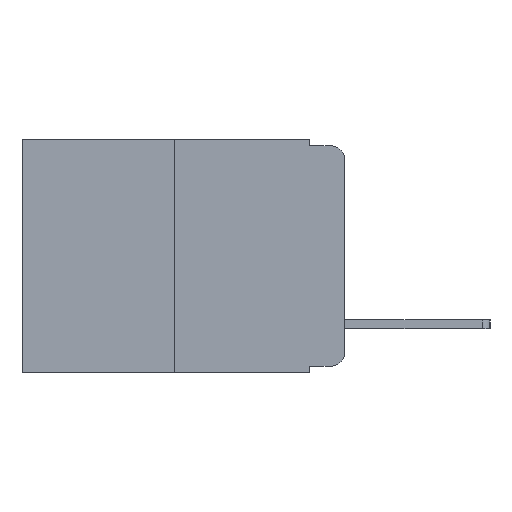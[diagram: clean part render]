
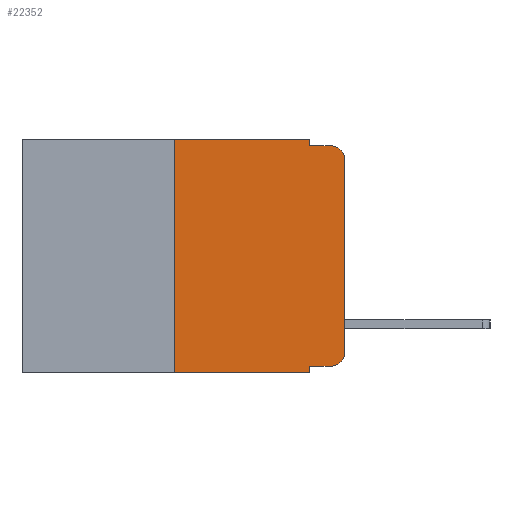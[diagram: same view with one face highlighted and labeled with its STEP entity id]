
A CAD part, left-side view. The second image highlights one B-rep face of the part: STEP entity #22352.
In plain terms, the highlighted planar face has unit normal (-1, 0, 0).
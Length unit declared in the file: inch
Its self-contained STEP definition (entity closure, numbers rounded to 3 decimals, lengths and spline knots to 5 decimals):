
#346 = CARTESIAN_POINT ( 'NONE',  ( 0., 0.051, -0.333 ) ) ;
#444 = CARTESIAN_POINT ( 'NONE',  ( 0., 0.02, -0.313 ) ) ;
#696 = EDGE_CURVE ( 'NONE', #20087, #22232, #1497, .T. ) ;
#750 = VERTEX_POINT ( 'NONE', #14333 ) ;
#879 = EDGE_CURVE ( 'NONE', #14549, #750, #12049, .T. ) ;
#1497 = LINE ( 'NONE', #20543, #21578 ) ;
#1663 = CARTESIAN_POINT ( 'NONE',  ( 0., 0.051, -0.01 ) ) ;
#2010 = EDGE_CURVE ( 'NONE', #13390, #22232, #22094, .T. ) ;
#2052 = VECTOR ( 'NONE', #11614, 39.37008 ) ;
#2058 = LINE ( 'NONE', #346, #11725 ) ;
#2358 = EDGE_CURVE ( 'NONE', #5249, #17747, #18879, .T. ) ;
#2439 = DIRECTION ( 'NONE',  ( 0., 0., -1. ) ) ;
#2460 = CARTESIAN_POINT ( 'NONE',  ( 0., 0.02, -0.03 ) ) ;
#3865 = DIRECTION ( 'NONE',  ( 0., -1., 0. ) ) ;
#4219 = ORIENTED_EDGE ( 'NONE', *, *, #10292, .T. ) ;
#4291 = ORIENTED_EDGE ( 'NONE', *, *, #14017, .T. ) ;
#4403 = DIRECTION ( 'NONE',  ( 0., -1., 0. ) ) ;
#4554 = CARTESIAN_POINT ( 'NONE',  ( 0., 0.051, -0.333 ) ) ;
#4584 = ORIENTED_EDGE ( 'NONE', *, *, #15250, .F. ) ;
#4840 = PLANE ( 'NONE',  #10993 ) ;
#5046 = VERTEX_POINT ( 'NONE', #6296 ) ;
#5072 = ORIENTED_EDGE ( 'NONE', *, *, #2358, .T. ) ;
#5108 = VECTOR ( 'NONE', #3865, 39.37008 ) ;
#5249 = VERTEX_POINT ( 'NONE', #21710 ) ;
#5967 = EDGE_CURVE ( 'NONE', #5046, #13390, #11704, .T. ) ;
#6157 = CARTESIAN_POINT ( 'NONE',  ( 0., 0.051, 0. ) ) ;
#6296 = CARTESIAN_POINT ( 'NONE',  ( 0., 0., -0.313 ) ) ;
#6336 = EDGE_LOOP ( 'NONE', ( #11376, #19580, #7520, #10325, #10302, #20525, #5072, #4584, #4291, #4219 ) ) ;
#6455 = DIRECTION ( 'NONE',  ( 0., 0., 1. ) ) ;
#6818 = CARTESIAN_POINT ( 'NONE',  ( 0., 0.473, 0. ) ) ;
#7274 = LINE ( 'NONE', #17069, #2052 ) ;
#7520 = ORIENTED_EDGE ( 'NONE', *, *, #696, .F. ) ;
#8120 = CARTESIAN_POINT ( 'NONE',  ( 0., 0.02, -0.333 ) ) ;
#8569 = CARTESIAN_POINT ( 'NONE',  ( 0., 0.051, -0.343 ) ) ;
#8710 = LINE ( 'NONE', #12100, #13090 ) ;
#8737 = DIRECTION ( 'NONE',  ( 0., 0., -1. ) ) ;
#9119 = AXIS2_PLACEMENT_3D ( 'NONE', #2460, #13047, #22651 ) ;
#9215 = VECTOR ( 'NONE', #10004, 39.37008 ) ;
#9375 = FACE_OUTER_BOUND ( 'NONE', #6336, .T. ) ;
#9574 = DIRECTION ( 'NONE',  ( 0., 0., 1. ) ) ;
#10004 = DIRECTION ( 'NONE',  ( 0., 0., -1. ) ) ;
#10292 = EDGE_CURVE ( 'NONE', #13618, #5046, #19519, .T. ) ;
#10302 = ORIENTED_EDGE ( 'NONE', *, *, #879, .F. ) ;
#10325 = ORIENTED_EDGE ( 'NONE', *, *, #22668, .F. ) ;
#10993 = AXIS2_PLACEMENT_3D ( 'NONE', #6818, #19822, #8737 ) ;
#11376 = ORIENTED_EDGE ( 'NONE', *, *, #5967, .T. ) ;
#11406 = AXIS2_PLACEMENT_3D ( 'NONE', #444, #13887, #2439 ) ;
#11614 = DIRECTION ( 'NONE',  ( 0., 0., -1. ) ) ;
#11704 = LINE ( 'NONE', #20640, #21499 ) ;
#11725 = VECTOR ( 'NONE', #17455, 39.37008 ) ;
#12049 = LINE ( 'NONE', #15333, #21270 ) ;
#12100 = CARTESIAN_POINT ( 'NONE',  ( 0., 0.25, 0. ) ) ;
#13047 = DIRECTION ( 'NONE',  ( -1., 0., 0. ) ) ;
#13082 = VERTEX_POINT ( 'NONE', #4554 ) ;
#13090 = VECTOR ( 'NONE', #6455, 39.37008 ) ;
#13390 = VERTEX_POINT ( 'NONE', #24149 ) ;
#13618 = VERTEX_POINT ( 'NONE', #8120 ) ;
#13887 = DIRECTION ( 'NONE',  ( -1., 0., 0. ) ) ;
#14017 = EDGE_CURVE ( 'NONE', #13082, #13618, #2058, .T. ) ;
#14162 = LINE ( 'NONE', #6157, #9215 ) ;
#14333 = CARTESIAN_POINT ( 'NONE',  ( 0., 0.051, 0. ) ) ;
#14549 = VERTEX_POINT ( 'NONE', #15274 ) ;
#15250 = EDGE_CURVE ( 'NONE', #13082, #17747, #14162, .T. ) ;
#15274 = CARTESIAN_POINT ( 'NONE',  ( 0., 0.25, 0. ) ) ;
#15333 = CARTESIAN_POINT ( 'NONE',  ( 0., 0.473, 0. ) ) ;
#17069 = CARTESIAN_POINT ( 'NONE',  ( 0., 0.051, 0. ) ) ;
#17455 = DIRECTION ( 'NONE',  ( 0., -1., 0. ) ) ;
#17705 = EDGE_CURVE ( 'NONE', #5249, #14549, #8710, .T. ) ;
#17747 = VERTEX_POINT ( 'NONE', #8569 ) ;
#18879 = LINE ( 'NONE', #22548, #5108 ) ;
#19519 = CIRCLE ( 'NONE', #11406, 0.02 ) ;
#19580 = ORIENTED_EDGE ( 'NONE', *, *, #2010, .T. ) ;
#19822 = DIRECTION ( 'NONE',  ( 1., 0., 0. ) ) ;
#20087 = VERTEX_POINT ( 'NONE', #1663 ) ;
#20525 = ORIENTED_EDGE ( 'NONE', *, *, #17705, .F. ) ;
#20543 = CARTESIAN_POINT ( 'NONE',  ( 0., 0.051, -0.01 ) ) ;
#20632 = DIRECTION ( 'NONE',  ( 0., -1., 0. ) ) ;
#20640 = CARTESIAN_POINT ( 'NONE',  ( 0., 0., 0. ) ) ;
#21202 = CARTESIAN_POINT ( 'NONE',  ( 0., 0.02, -0.01 ) ) ;
#21270 = VECTOR ( 'NONE', #4403, 39.37008 ) ;
#21499 = VECTOR ( 'NONE', #9574, 39.37008 ) ;
#21578 = VECTOR ( 'NONE', #20632, 39.37008 ) ;
#21710 = CARTESIAN_POINT ( 'NONE',  ( 0., 0.25, -0.343 ) ) ;
#22094 = CIRCLE ( 'NONE', #9119, 0.02 ) ;
#22232 = VERTEX_POINT ( 'NONE', #21202 ) ;
#22352 = ADVANCED_FACE ( 'NONE', ( #9375 ), #4840, .F. ) ;
#22548 = CARTESIAN_POINT ( 'NONE',  ( 0., 0.473, -0.343 ) ) ;
#22651 = DIRECTION ( 'NONE',  ( 0., 0., -1. ) ) ;
#22668 = EDGE_CURVE ( 'NONE', #750, #20087, #7274, .T. ) ;
#24149 = CARTESIAN_POINT ( 'NONE',  ( 0., 0., -0.03 ) ) ;
